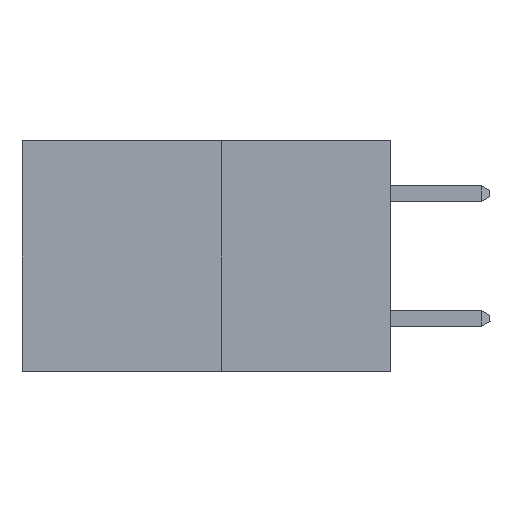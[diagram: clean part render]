
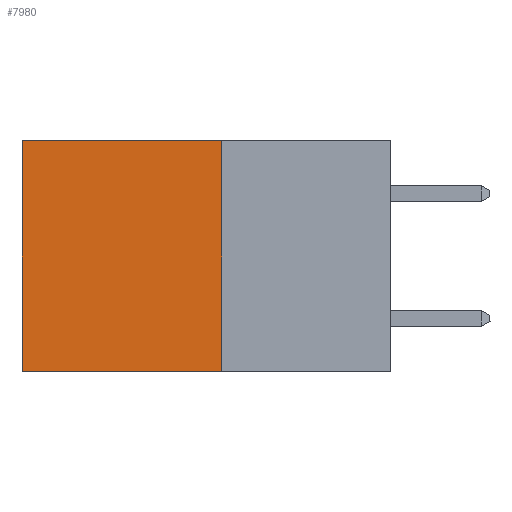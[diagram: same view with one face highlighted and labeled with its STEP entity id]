
A CAD part, left-side view. The second image highlights one B-rep face of the part: STEP entity #7980.
In plain terms, the highlighted planar face has unit normal (-1, 0, 0).
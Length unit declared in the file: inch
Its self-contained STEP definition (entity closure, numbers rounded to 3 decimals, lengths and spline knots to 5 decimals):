
#186 = CARTESIAN_POINT ( 'NONE',  ( 0.277, 0.59, 0. ) ) ;
#378 = AXIS2_PLACEMENT_3D ( 'NONE', #751, #745, #675 ) ;
#427 = ORIENTED_EDGE ( 'NONE', *, *, #9190, .F. ) ;
#675 = DIRECTION ( 'NONE',  ( 0., 0., -1. ) ) ;
#745 = DIRECTION ( 'NONE',  ( 1., 0., 0. ) ) ;
#751 = CARTESIAN_POINT ( 'NONE',  ( 0.277, 0.27, -0.37 ) ) ;
#781 = PLANE ( 'NONE',  #378 ) ;
#858 = CARTESIAN_POINT ( 'NONE',  ( 0.277, 0.59, -0.37 ) ) ;
#1526 = VECTOR ( 'NONE', #2708, 39.37008 ) ;
#1725 = LINE ( 'NONE', #2136, #10194 ) ;
#2136 = CARTESIAN_POINT ( 'NONE',  ( 0.277, 0.27, -0.37 ) ) ;
#2305 = CARTESIAN_POINT ( 'NONE',  ( 0.277, 0.27, -0.37 ) ) ;
#2708 = DIRECTION ( 'NONE',  ( 0., 0., -1. ) ) ;
#4010 = CARTESIAN_POINT ( 'NONE',  ( 0.277, 0.27, -0.37 ) ) ;
#4387 = VERTEX_POINT ( 'NONE', #858 ) ;
#5024 = ORIENTED_EDGE ( 'NONE', *, *, #8247, .T. ) ;
#7228 = DIRECTION ( 'NONE',  ( 0., 1., 0. ) ) ;
#7472 = CARTESIAN_POINT ( 'NONE',  ( 0.277, 0.27, 0. ) ) ;
#7668 = CARTESIAN_POINT ( 'NONE',  ( 0.277, 0.27, 0. ) ) ;
#7855 = VERTEX_POINT ( 'NONE', #2305 ) ;
#7980 = ADVANCED_FACE ( 'NONE', ( #21737 ), #781, .F. ) ;
#8241 = LINE ( 'NONE', #7472, #19930 ) ;
#8247 = EDGE_CURVE ( 'NONE', #10778, #21178, #8241, .T. ) ;
#9190 = EDGE_CURVE ( 'NONE', #10778, #7855, #11059, .T. ) ;
#10194 = VECTOR ( 'NONE', #10627, 39.37008 ) ;
#10627 = DIRECTION ( 'NONE',  ( 0., 1., 0. ) ) ;
#10778 = VERTEX_POINT ( 'NONE', #7668 ) ;
#11059 = LINE ( 'NONE', #4010, #1526 ) ;
#11219 = CARTESIAN_POINT ( 'NONE',  ( 0.277, 0.59, -0.37 ) ) ;
#11330 = EDGE_LOOP ( 'NONE', ( #17563, #19672, #427, #5024 ) ) ;
#14367 = VECTOR ( 'NONE', #21158, 39.37008 ) ;
#17563 = ORIENTED_EDGE ( 'NONE', *, *, #18355, .T. ) ;
#18112 = EDGE_CURVE ( 'NONE', #7855, #4387, #1725, .T. ) ;
#18355 = EDGE_CURVE ( 'NONE', #21178, #4387, #19293, .T. ) ;
#19293 = LINE ( 'NONE', #11219, #14367 ) ;
#19672 = ORIENTED_EDGE ( 'NONE', *, *, #18112, .F. ) ;
#19930 = VECTOR ( 'NONE', #7228, 39.37008 ) ;
#21158 = DIRECTION ( 'NONE',  ( 0., 0., -1. ) ) ;
#21178 = VERTEX_POINT ( 'NONE', #186 ) ;
#21737 = FACE_OUTER_BOUND ( 'NONE', #11330, .T. ) ;
